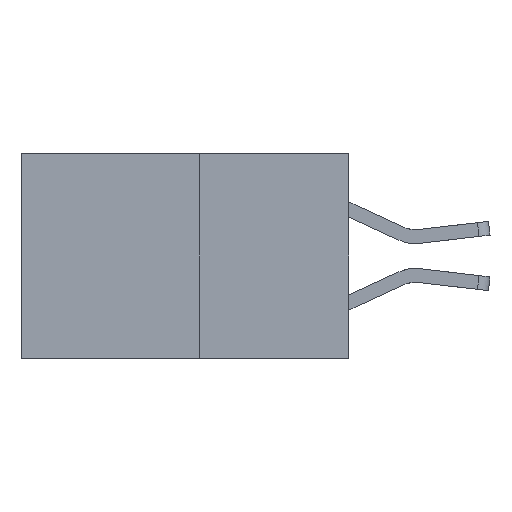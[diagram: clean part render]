
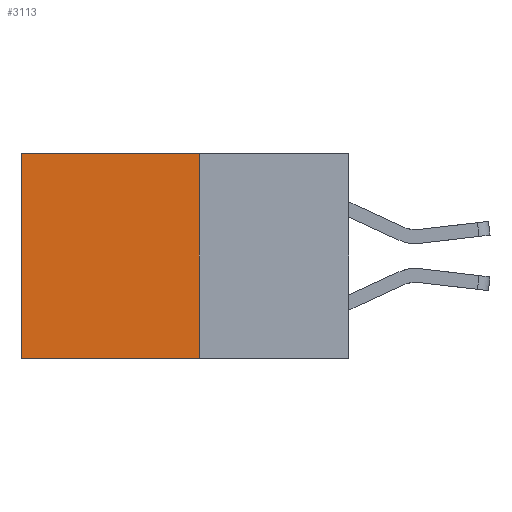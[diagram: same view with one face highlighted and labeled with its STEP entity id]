
A CAD part, left-side view. The second image highlights one B-rep face of the part: STEP entity #3113.
In plain terms, the highlighted planar face has unit normal (-1, 0, 0).
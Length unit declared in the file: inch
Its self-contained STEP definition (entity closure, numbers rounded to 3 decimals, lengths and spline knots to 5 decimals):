
#586 = FACE_OUTER_BOUND ( 'NONE', #2177, .T. ) ;
#685 = LINE ( 'NONE', #10706, #5858 ) ;
#693 = AXIS2_PLACEMENT_3D ( 'NONE', #6148, #6093, #6090 ) ;
#1495 = EDGE_CURVE ( 'NONE', #8847, #9576, #685, .T. ) ;
#1677 = VECTOR ( 'NONE', #12053, 39.37008 ) ;
#1986 = LINE ( 'NONE', #4374, #7079 ) ;
#2177 = EDGE_LOOP ( 'NONE', ( #11296, #6054, #6293, #10043 ) ) ;
#2779 = VERTEX_POINT ( 'NONE', #8260 ) ;
#2863 = VERTEX_POINT ( 'NONE', #7569 ) ;
#3113 = ADVANCED_FACE ( 'NONE', ( #586 ), #6224, .F. ) ;
#4051 = CARTESIAN_POINT ( 'NONE',  ( 0.277, 0.27, -0.37 ) ) ;
#4374 = CARTESIAN_POINT ( 'NONE',  ( 0.277, 0.27, -0.37 ) ) ;
#4982 = EDGE_CURVE ( 'NONE', #9576, #2779, #5887, .T. ) ;
#5097 = CARTESIAN_POINT ( 'NONE',  ( 0.277, 0.59, 0. ) ) ;
#5468 = DIRECTION ( 'NONE',  ( 0., 0., -1. ) ) ;
#5481 = CARTESIAN_POINT ( 'NONE',  ( 0.277, 0.59, -0.37 ) ) ;
#5858 = VECTOR ( 'NONE', #11104, 39.37008 ) ;
#5887 = LINE ( 'NONE', #5481, #8514 ) ;
#6054 = ORIENTED_EDGE ( 'NONE', *, *, #10291, .F. ) ;
#6090 = DIRECTION ( 'NONE',  ( 0., 0., -1. ) ) ;
#6093 = DIRECTION ( 'NONE',  ( 1., 0., 0. ) ) ;
#6148 = CARTESIAN_POINT ( 'NONE',  ( 0.277, 0.27, -0.37 ) ) ;
#6224 = PLANE ( 'NONE',  #693 ) ;
#6227 = EDGE_CURVE ( 'NONE', #8847, #2863, #1986, .T. ) ;
#6293 = ORIENTED_EDGE ( 'NONE', *, *, #6227, .F. ) ;
#6827 = CARTESIAN_POINT ( 'NONE',  ( 0.277, 0.27, 0. ) ) ;
#7079 = VECTOR ( 'NONE', #9474, 39.37008 ) ;
#7084 = LINE ( 'NONE', #4051, #1677 ) ;
#7569 = CARTESIAN_POINT ( 'NONE',  ( 0.277, 0.27, -0.37 ) ) ;
#8260 = CARTESIAN_POINT ( 'NONE',  ( 0.277, 0.59, -0.37 ) ) ;
#8514 = VECTOR ( 'NONE', #5468, 39.37008 ) ;
#8847 = VERTEX_POINT ( 'NONE', #6827 ) ;
#9474 = DIRECTION ( 'NONE',  ( 0., 0., -1. ) ) ;
#9576 = VERTEX_POINT ( 'NONE', #5097 ) ;
#10043 = ORIENTED_EDGE ( 'NONE', *, *, #1495, .T. ) ;
#10291 = EDGE_CURVE ( 'NONE', #2863, #2779, #7084, .T. ) ;
#10706 = CARTESIAN_POINT ( 'NONE',  ( 0.277, 0.27, 0. ) ) ;
#11104 = DIRECTION ( 'NONE',  ( 0., 1., 0. ) ) ;
#11296 = ORIENTED_EDGE ( 'NONE', *, *, #4982, .T. ) ;
#12053 = DIRECTION ( 'NONE',  ( 0., 1., 0. ) ) ;
